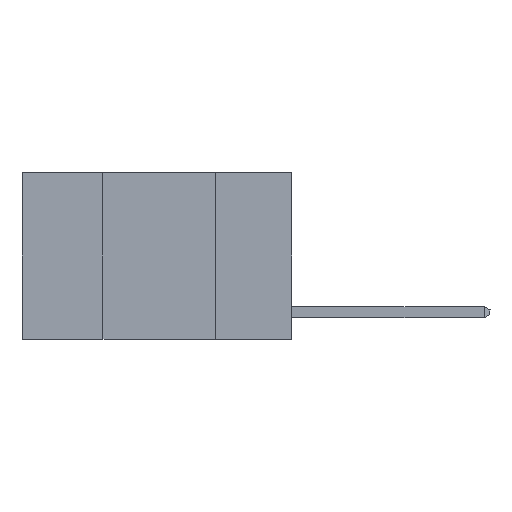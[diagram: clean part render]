
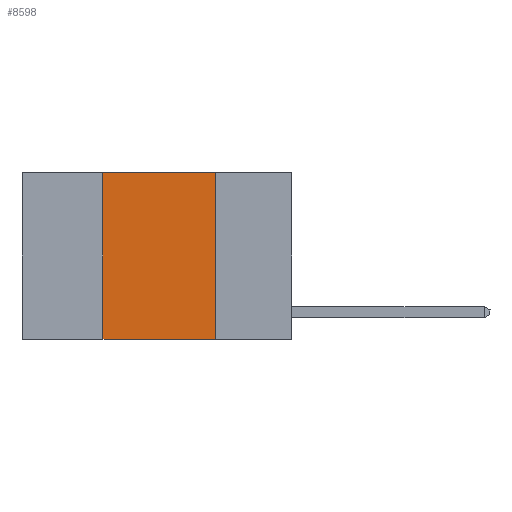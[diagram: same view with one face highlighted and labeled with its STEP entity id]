
A CAD part, left-side view. The second image highlights one B-rep face of the part: STEP entity #8598.
In plain terms, the highlighted planar face has unit normal (-1, 0, 0).
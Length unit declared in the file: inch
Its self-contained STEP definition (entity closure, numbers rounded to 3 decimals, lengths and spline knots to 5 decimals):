
#1454 = AXIS2_PLACEMENT_3D ( 'NONE', #17093, #13980, #14172 ) ;
#1556 = EDGE_CURVE ( 'NONE', #18193, #18830, #12795, .T. ) ;
#1773 = ORIENTED_EDGE ( 'NONE', *, *, #13362, .T. ) ;
#2148 = DIRECTION ( 'NONE',  ( 0., 0., 1. ) ) ;
#3304 = VECTOR ( 'NONE', #2148, 39.37008 ) ;
#3871 = ORIENTED_EDGE ( 'NONE', *, *, #1556, .F. ) ;
#4864 = EDGE_CURVE ( 'NONE', #18830, #17016, #6829, .T. ) ;
#5020 = DIRECTION ( 'NONE',  ( 0., -1., 0. ) ) ;
#5344 = DIRECTION ( 'NONE',  ( 0., -1., 0. ) ) ;
#5427 = EDGE_LOOP ( 'NONE', ( #14907, #18796, #3871, #1773 ) ) ;
#5973 = CARTESIAN_POINT ( 'NONE',  ( 0., 0.42, -0.37 ) ) ;
#6829 = LINE ( 'NONE', #18626, #9354 ) ;
#7306 = VECTOR ( 'NONE', #5020, 39.37008 ) ;
#8155 = LINE ( 'NONE', #11032, #7306 ) ;
#8369 = VECTOR ( 'NONE', #10419, 39.37008 ) ;
#8598 = ADVANCED_FACE ( 'NONE', ( #13886 ), #15609, .F. ) ;
#9354 = VECTOR ( 'NONE', #5344, 39.37008 ) ;
#9546 = VERTEX_POINT ( 'NONE', #14012 ) ;
#10419 = DIRECTION ( 'NONE',  ( 0., 0., -1. ) ) ;
#10692 = CARTESIAN_POINT ( 'NONE',  ( 0., 0.17, 0. ) ) ;
#11032 = CARTESIAN_POINT ( 'NONE',  ( 0., 0.6, -0.37 ) ) ;
#11077 = EDGE_CURVE ( 'NONE', #17016, #9546, #12049, .T. ) ;
#12049 = LINE ( 'NONE', #10692, #8369 ) ;
#12795 = LINE ( 'NONE', #15417, #3304 ) ;
#13362 = EDGE_CURVE ( 'NONE', #18193, #9546, #8155, .T. ) ;
#13886 = FACE_OUTER_BOUND ( 'NONE', #5427, .T. ) ;
#13980 = DIRECTION ( 'NONE',  ( 1., 0., 0. ) ) ;
#14012 = CARTESIAN_POINT ( 'NONE',  ( 0., 0.17, -0.37 ) ) ;
#14172 = DIRECTION ( 'NONE',  ( 0., 0., -1. ) ) ;
#14907 = ORIENTED_EDGE ( 'NONE', *, *, #11077, .F. ) ;
#15417 = CARTESIAN_POINT ( 'NONE',  ( 0., 0.42, 0. ) ) ;
#15609 = PLANE ( 'NONE',  #1454 ) ;
#16229 = CARTESIAN_POINT ( 'NONE',  ( 0., 0.42, 0. ) ) ;
#17016 = VERTEX_POINT ( 'NONE', #17410 ) ;
#17093 = CARTESIAN_POINT ( 'NONE',  ( 0., 0.6, 0. ) ) ;
#17410 = CARTESIAN_POINT ( 'NONE',  ( 0., 0.17, 0. ) ) ;
#18193 = VERTEX_POINT ( 'NONE', #5973 ) ;
#18626 = CARTESIAN_POINT ( 'NONE',  ( 0., 0.6, 0. ) ) ;
#18796 = ORIENTED_EDGE ( 'NONE', *, *, #4864, .F. ) ;
#18830 = VERTEX_POINT ( 'NONE', #16229 ) ;
